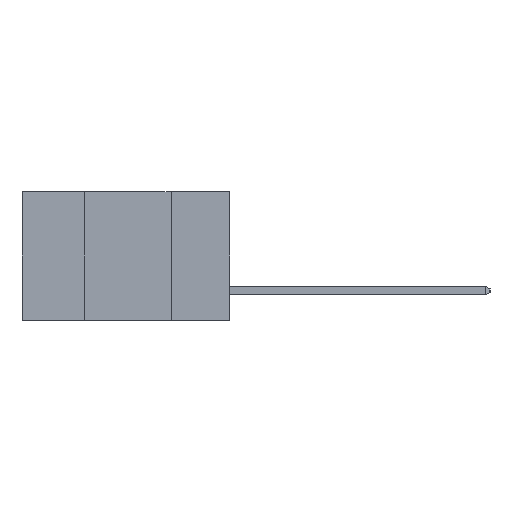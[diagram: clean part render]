
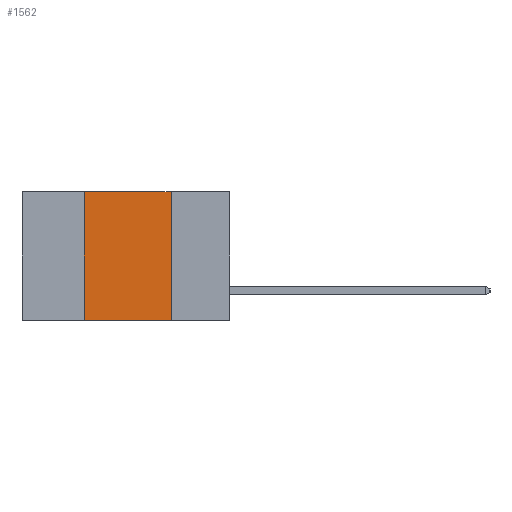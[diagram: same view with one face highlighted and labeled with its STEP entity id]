
A CAD part, left-side view. The second image highlights one B-rep face of the part: STEP entity #1562.
In plain terms, the highlighted planar face has unit normal (-1, 0, 0).
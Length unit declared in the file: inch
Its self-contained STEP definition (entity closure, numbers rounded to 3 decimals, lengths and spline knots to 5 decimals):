
#307 = VECTOR ( 'NONE', #6159, 39.37008 ) ;
#412 = DIRECTION ( 'NONE',  ( 1., 0., 0. ) ) ;
#451 = PLANE ( 'NONE',  #5124 ) ;
#1230 = CARTESIAN_POINT ( 'NONE',  ( 0., 0.42, -0.37 ) ) ;
#1478 = EDGE_CURVE ( 'NONE', #3801, #10049, #3305, .T. ) ;
#1562 = ADVANCED_FACE ( 'NONE', ( #12806 ), #451, .F. ) ;
#1938 = CARTESIAN_POINT ( 'NONE',  ( 0., 0.17, -0.37 ) ) ;
#2216 = EDGE_CURVE ( 'NONE', #3801, #3113, #8423, .T. ) ;
#2238 = CARTESIAN_POINT ( 'NONE',  ( 0., 0.6, 0. ) ) ;
#2291 = DIRECTION ( 'NONE',  ( 0., -1., 0. ) ) ;
#2314 = DIRECTION ( 'NONE',  ( 0., 0., -1. ) ) ;
#2973 = DIRECTION ( 'NONE',  ( 0., 0., 1. ) ) ;
#2974 = EDGE_CURVE ( 'NONE', #3113, #5981, #7932, .T. ) ;
#3113 = VERTEX_POINT ( 'NONE', #9402 ) ;
#3199 = CARTESIAN_POINT ( 'NONE',  ( 0., 0.42, -0.37 ) ) ;
#3270 = LINE ( 'NONE', #1938, #307 ) ;
#3305 = LINE ( 'NONE', #5692, #10957 ) ;
#3310 = VECTOR ( 'NONE', #2973, 39.37008 ) ;
#3538 = ORIENTED_EDGE ( 'NONE', *, *, #11228, .F. ) ;
#3655 = EDGE_LOOP ( 'NONE', ( #3538, #8613, #5965, #10869 ) ) ;
#3801 = VERTEX_POINT ( 'NONE', #1230 ) ;
#5124 = AXIS2_PLACEMENT_3D ( 'NONE', #5603, #412, #2314 ) ;
#5252 = VECTOR ( 'NONE', #2291, 39.37008 ) ;
#5416 = DIRECTION ( 'NONE',  ( 0., -1., 0. ) ) ;
#5603 = CARTESIAN_POINT ( 'NONE',  ( 0., 0.6, 0. ) ) ;
#5692 = CARTESIAN_POINT ( 'NONE',  ( 0., 0.6, -0.37 ) ) ;
#5965 = ORIENTED_EDGE ( 'NONE', *, *, #2216, .F. ) ;
#5981 = VERTEX_POINT ( 'NONE', #10899 ) ;
#6159 = DIRECTION ( 'NONE',  ( 0., 0., -1. ) ) ;
#7369 = CARTESIAN_POINT ( 'NONE',  ( 0., 0.17, -0.37 ) ) ;
#7932 = LINE ( 'NONE', #2238, #5252 ) ;
#8423 = LINE ( 'NONE', #3199, #3310 ) ;
#8613 = ORIENTED_EDGE ( 'NONE', *, *, #2974, .F. ) ;
#9402 = CARTESIAN_POINT ( 'NONE',  ( 0., 0.42, 0. ) ) ;
#10049 = VERTEX_POINT ( 'NONE', #7369 ) ;
#10869 = ORIENTED_EDGE ( 'NONE', *, *, #1478, .T. ) ;
#10899 = CARTESIAN_POINT ( 'NONE',  ( 0., 0.17, 0. ) ) ;
#10957 = VECTOR ( 'NONE', #5416, 39.37008 ) ;
#11228 = EDGE_CURVE ( 'NONE', #5981, #10049, #3270, .T. ) ;
#12806 = FACE_OUTER_BOUND ( 'NONE', #3655, .T. ) ;
